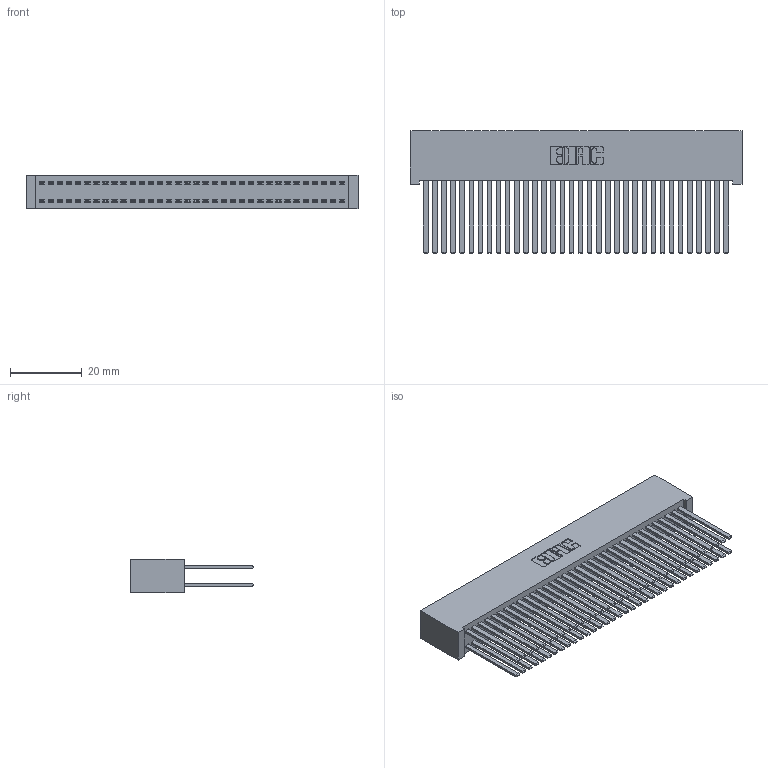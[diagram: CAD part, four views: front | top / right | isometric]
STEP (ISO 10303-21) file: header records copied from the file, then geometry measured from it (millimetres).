
FILE_DESCRIPTION (( 'STEP AP203' ), '1' );
FILE_NAME ('392-068-544-201.STEP', '2019-10-09T11:42:38', ( '' ), ( '' ), 'SwSTEP 2.0', 'SolidWorks 2016', '' );
FILE_SCHEMA (( 'CONFIG_CONTROL_DESIGN' ));
Length unit declared in the file: inch
Products named in the file (3): 345-292-001_345-293-144; 392-068-544-201; 342 Part_Lugless
Assembly tree (69 placements, depth 2):
  392-068-544-201
    342 Part_Lugless
    345-292-001_345-293-144  x68
Bounding box: 92.61 x 34.3 x 9.4 mm (x, y, z)
Volume: 9675.7 mm3; surface area: 18638.6 mm2
Topology: 69 solids, 69 shells, 3230 faces, 9591 edges, 6302 vertices
Faces by surface type: plane 2238, cylinder 992
Entity records: 22315 total; most frequent: CARTESIAN_POINT 3702, ORIENTED_EDGE 3638, DIRECTION 3167, EDGE_CURVE 1819, VECTOR 1703, LINE 1703, VERTEX_POINT 1210, AXIS2_PLACEMENT_3D 732
